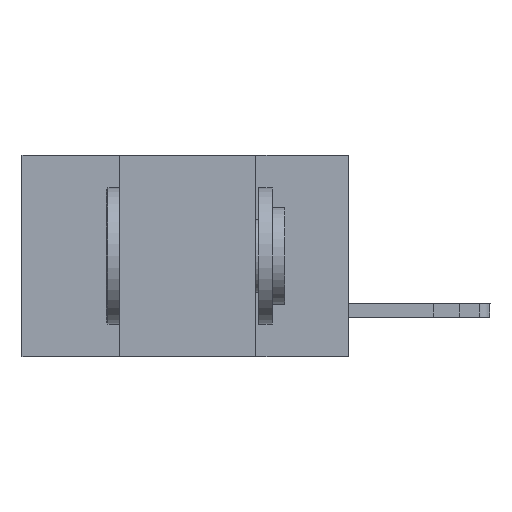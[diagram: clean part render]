
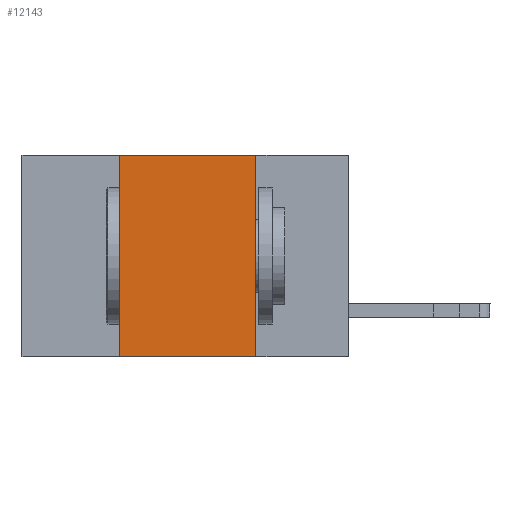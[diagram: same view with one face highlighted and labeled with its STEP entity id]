
A CAD part, left-side view. The second image highlights one B-rep face of the part: STEP entity #12143.
In plain terms, the highlighted planar face has unit normal (-1, 0, 0).
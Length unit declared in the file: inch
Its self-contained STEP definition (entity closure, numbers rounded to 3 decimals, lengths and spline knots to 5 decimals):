
#266 = CARTESIAN_POINT ( 'NONE',  ( 0., 0.6, 0. ) ) ;
#410 = DIRECTION ( 'NONE',  ( 0., -1., 0. ) ) ;
#421 = CARTESIAN_POINT ( 'NONE',  ( 0., 0.42, -0.37 ) ) ;
#1308 = DIRECTION ( 'NONE',  ( 0., 0., -1. ) ) ;
#1607 = PLANE ( 'NONE',  #5055 ) ;
#1805 = DIRECTION ( 'NONE',  ( 0., 0., 1. ) ) ;
#2636 = VERTEX_POINT ( 'NONE', #12599 ) ;
#2957 = DIRECTION ( 'NONE',  ( 0., 0., -1. ) ) ;
#4068 = LINE ( 'NONE', #421, #9561 ) ;
#4213 = VECTOR ( 'NONE', #1308, 39.37008 ) ;
#4647 = CARTESIAN_POINT ( 'NONE',  ( 0., 0.17, -0.37 ) ) ;
#5055 = AXIS2_PLACEMENT_3D ( 'NONE', #8362, #11035, #2957 ) ;
#5605 = EDGE_CURVE ( 'NONE', #14180, #6310, #7639, .T. ) ;
#6310 = VERTEX_POINT ( 'NONE', #4647 ) ;
#6380 = VECTOR ( 'NONE', #10606, 39.37008 ) ;
#7435 = EDGE_CURVE ( 'NONE', #2636, #17221, #12643, .T. ) ;
#7639 = LINE ( 'NONE', #10601, #6380 ) ;
#7686 = ORIENTED_EDGE ( 'NONE', *, *, #8828, .F. ) ;
#8362 = CARTESIAN_POINT ( 'NONE',  ( 0., 0.6, 0. ) ) ;
#8828 = EDGE_CURVE ( 'NONE', #17221, #6310, #14831, .T. ) ;
#9561 = VECTOR ( 'NONE', #1805, 39.37008 ) ;
#10601 = CARTESIAN_POINT ( 'NONE',  ( 0., 0.6, -0.37 ) ) ;
#10606 = DIRECTION ( 'NONE',  ( 0., -1., 0. ) ) ;
#11035 = DIRECTION ( 'NONE',  ( 1., 0., 0. ) ) ;
#11037 = ORIENTED_EDGE ( 'NONE', *, *, #7435, .F. ) ;
#12143 = ADVANCED_FACE ( 'NONE', ( #15432 ), #1607, .F. ) ;
#12599 = CARTESIAN_POINT ( 'NONE',  ( 0., 0.42, 0. ) ) ;
#12643 = LINE ( 'NONE', #266, #13056 ) ;
#12901 = CARTESIAN_POINT ( 'NONE',  ( 0., 0.17, 0. ) ) ;
#13056 = VECTOR ( 'NONE', #410, 39.37008 ) ;
#13686 = ORIENTED_EDGE ( 'NONE', *, *, #16520, .F. ) ;
#14180 = VERTEX_POINT ( 'NONE', #17085 ) ;
#14622 = EDGE_LOOP ( 'NONE', ( #7686, #11037, #13686, #16498 ) ) ;
#14831 = LINE ( 'NONE', #17172, #4213 ) ;
#15432 = FACE_OUTER_BOUND ( 'NONE', #14622, .T. ) ;
#16498 = ORIENTED_EDGE ( 'NONE', *, *, #5605, .T. ) ;
#16520 = EDGE_CURVE ( 'NONE', #14180, #2636, #4068, .T. ) ;
#17085 = CARTESIAN_POINT ( 'NONE',  ( 0., 0.42, -0.37 ) ) ;
#17172 = CARTESIAN_POINT ( 'NONE',  ( 0., 0.17, -0.37 ) ) ;
#17221 = VERTEX_POINT ( 'NONE', #12901 ) ;
